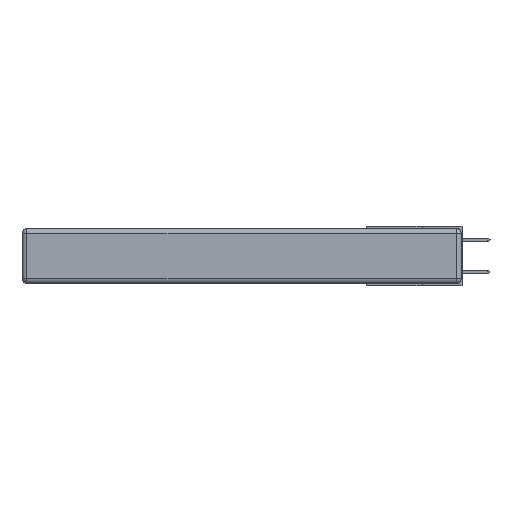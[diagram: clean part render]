
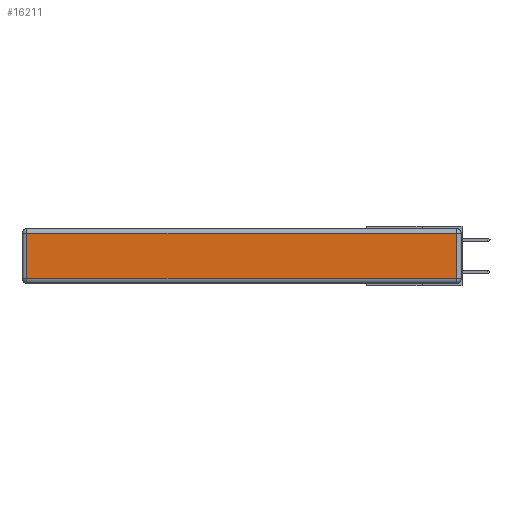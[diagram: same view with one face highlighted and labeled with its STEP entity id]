
A CAD part, left-side view. The second image highlights one B-rep face of the part: STEP entity #16211.
In plain terms, the highlighted planar face has unit normal (-1, 0, 0).
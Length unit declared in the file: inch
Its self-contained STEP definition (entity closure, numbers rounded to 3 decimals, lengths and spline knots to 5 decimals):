
#1084 = EDGE_LOOP ( 'NONE', ( #4893, #16372, #7560, #21500 ) ) ;
#2243 = CARTESIAN_POINT ( 'NONE',  ( 0., 2.72, -0.03 ) ) ;
#2643 = VERTEX_POINT ( 'NONE', #2243 ) ;
#3059 = DIRECTION ( 'NONE',  ( -1., 0., 0. ) ) ;
#3465 = LINE ( 'NONE', #11810, #25487 ) ;
#3640 = FACE_OUTER_BOUND ( 'NONE', #1084, .T. ) ;
#3706 = CARTESIAN_POINT ( 'NONE',  ( 0., 0., -0.313 ) ) ;
#3719 = DIRECTION ( 'NONE',  ( 0., 0., 1. ) ) ;
#4893 = ORIENTED_EDGE ( 'NONE', *, *, #15735, .T. ) ;
#5383 = DIRECTION ( 'NONE',  ( 0., 0., 1. ) ) ;
#5397 = DIRECTION ( 'NONE',  ( 0., 1., 0. ) ) ;
#6175 = LINE ( 'NONE', #3706, #14174 ) ;
#6619 = CARTESIAN_POINT ( 'NONE',  ( 0., 0.03, -0.03 ) ) ;
#7560 = ORIENTED_EDGE ( 'NONE', *, *, #21748, .T. ) ;
#10369 = LINE ( 'NONE', #27144, #14071 ) ;
#10584 = EDGE_CURVE ( 'NONE', #17637, #10981, #10369, .T. ) ;
#10642 = AXIS2_PLACEMENT_3D ( 'NONE', #13698, #3059, #5383 ) ;
#10981 = VERTEX_POINT ( 'NONE', #6619 ) ;
#11810 = CARTESIAN_POINT ( 'NONE',  ( 0., 2.75, -0.03 ) ) ;
#13582 = CARTESIAN_POINT ( 'NONE',  ( 0., 2.72, -0.343 ) ) ;
#13698 = CARTESIAN_POINT ( 'NONE',  ( 0., 0., -0.343 ) ) ;
#14071 = VECTOR ( 'NONE', #3719, 39.37008 ) ;
#14174 = VECTOR ( 'NONE', #20480, 39.37008 ) ;
#15735 = EDGE_CURVE ( 'NONE', #19788, #17637, #6175, .T. ) ;
#15745 = DIRECTION ( 'NONE',  ( 0., 0., -1. ) ) ;
#16211 = ADVANCED_FACE ( 'NONE', ( #3640 ), #24411, .T. ) ;
#16372 = ORIENTED_EDGE ( 'NONE', *, *, #10584, .T. ) ;
#17637 = VERTEX_POINT ( 'NONE', #27605 ) ;
#19788 = VERTEX_POINT ( 'NONE', #23829 ) ;
#19875 = LINE ( 'NONE', #13582, #22238 ) ;
#20480 = DIRECTION ( 'NONE',  ( 0., -1., 0. ) ) ;
#21500 = ORIENTED_EDGE ( 'NONE', *, *, #23381, .T. ) ;
#21748 = EDGE_CURVE ( 'NONE', #10981, #2643, #3465, .T. ) ;
#22238 = VECTOR ( 'NONE', #15745, 39.37008 ) ;
#23381 = EDGE_CURVE ( 'NONE', #2643, #19788, #19875, .T. ) ;
#23829 = CARTESIAN_POINT ( 'NONE',  ( 0., 2.72, -0.313 ) ) ;
#24411 = PLANE ( 'NONE',  #10642 ) ;
#25487 = VECTOR ( 'NONE', #5397, 39.37008 ) ;
#27144 = CARTESIAN_POINT ( 'NONE',  ( 0., 0.03, -0.343 ) ) ;
#27605 = CARTESIAN_POINT ( 'NONE',  ( 0., 0.03, -0.313 ) ) ;
